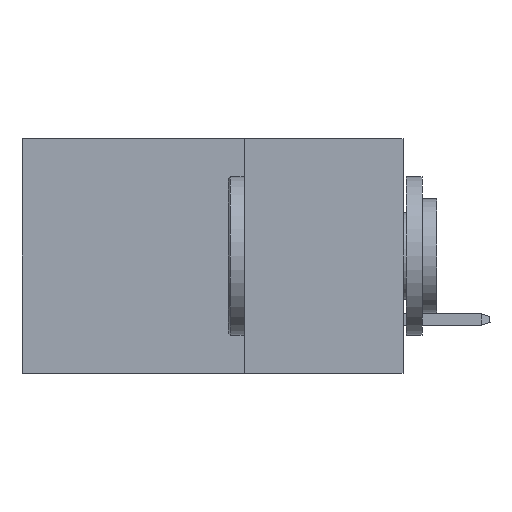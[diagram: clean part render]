
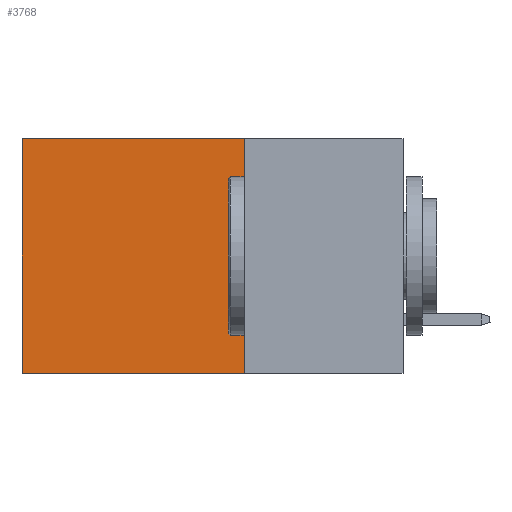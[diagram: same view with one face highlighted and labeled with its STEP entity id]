
A CAD part, left-side view. The second image highlights one B-rep face of the part: STEP entity #3768.
In plain terms, the highlighted planar face has unit normal (-1, 0, 0).
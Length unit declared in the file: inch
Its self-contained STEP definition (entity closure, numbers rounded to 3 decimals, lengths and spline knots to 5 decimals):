
#1 = VECTOR ( 'NONE', #4280, 39.37008 ) ;
#85 = DIRECTION ( 'NONE',  ( 0., 0., -1. ) ) ;
#1337 = CARTESIAN_POINT ( 'NONE',  ( 0.2875, 0.6, 0. ) ) ;
#1384 = CARTESIAN_POINT ( 'NONE',  ( 0.2875, 0.25, 0. ) ) ;
#1972 = CARTESIAN_POINT ( 'NONE',  ( 0.2875, 0.25, -0.37 ) ) ;
#3768 = ADVANCED_FACE ( 'NONE', ( #14108 ), #26371, .F. ) ;
#4280 = DIRECTION ( 'NONE',  ( 0., 0., -1. ) ) ;
#5163 = EDGE_CURVE ( 'NONE', #20608, #12332, #27541, .T. ) ;
#5285 = CARTESIAN_POINT ( 'NONE',  ( 0.2875, 0.25, 0. ) ) ;
#5823 = LINE ( 'NONE', #8714, #15570 ) ;
#6874 = ORIENTED_EDGE ( 'NONE', *, *, #5163, .F. ) ;
#7014 = CARTESIAN_POINT ( 'NONE',  ( 0.2875, 0.6, -0.37 ) ) ;
#7232 = VERTEX_POINT ( 'NONE', #15382 ) ;
#7665 = VECTOR ( 'NONE', #8379, 39.37008 ) ;
#8077 = DIRECTION ( 'NONE',  ( 1., 0., 0. ) ) ;
#8379 = DIRECTION ( 'NONE',  ( 0., 1., 0. ) ) ;
#8714 = CARTESIAN_POINT ( 'NONE',  ( 0.2875, 0.25, -0.37 ) ) ;
#10358 = ORIENTED_EDGE ( 'NONE', *, *, #30665, .T. ) ;
#12332 = VERTEX_POINT ( 'NONE', #1972 ) ;
#12641 = LINE ( 'NONE', #1337, #1 ) ;
#14108 = FACE_OUTER_BOUND ( 'NONE', #31370, .T. ) ;
#15382 = CARTESIAN_POINT ( 'NONE',  ( 0.2875, 0.6, 0. ) ) ;
#15570 = VECTOR ( 'NONE', #29564, 39.37008 ) ;
#19683 = LINE ( 'NONE', #5285, #7665 ) ;
#20304 = VECTOR ( 'NONE', #24642, 39.37008 ) ;
#20608 = VERTEX_POINT ( 'NONE', #1384 ) ;
#21058 = EDGE_CURVE ( 'NONE', #7232, #21170, #12641, .T. ) ;
#21170 = VERTEX_POINT ( 'NONE', #7014 ) ;
#21416 = EDGE_CURVE ( 'NONE', #12332, #21170, #5823, .T. ) ;
#22082 = ORIENTED_EDGE ( 'NONE', *, *, #21058, .T. ) ;
#24642 = DIRECTION ( 'NONE',  ( 0., 0., -1. ) ) ;
#26371 = PLANE ( 'NONE',  #38261 ) ;
#27541 = LINE ( 'NONE', #30085, #20304 ) ;
#29218 = ORIENTED_EDGE ( 'NONE', *, *, #21416, .F. ) ;
#29564 = DIRECTION ( 'NONE',  ( 0., 1., 0. ) ) ;
#30085 = CARTESIAN_POINT ( 'NONE',  ( 0.2875, 0.25, 0. ) ) ;
#30665 = EDGE_CURVE ( 'NONE', #20608, #7232, #19683, .T. ) ;
#31370 = EDGE_LOOP ( 'NONE', ( #22082, #29218, #6874, #10358 ) ) ;
#32413 = CARTESIAN_POINT ( 'NONE',  ( 0.2875, 0.25, 0. ) ) ;
#38261 = AXIS2_PLACEMENT_3D ( 'NONE', #32413, #8077, #85 ) ;
